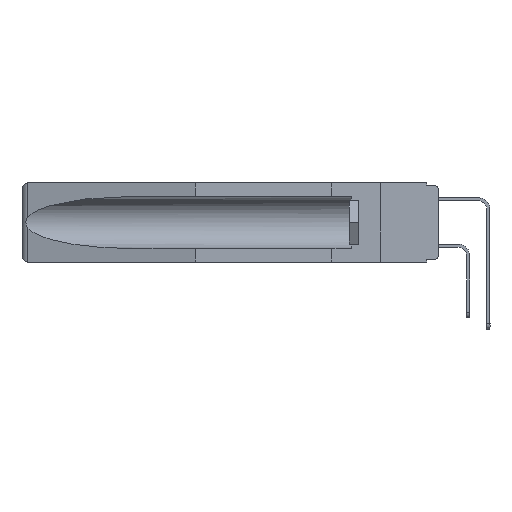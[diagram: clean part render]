
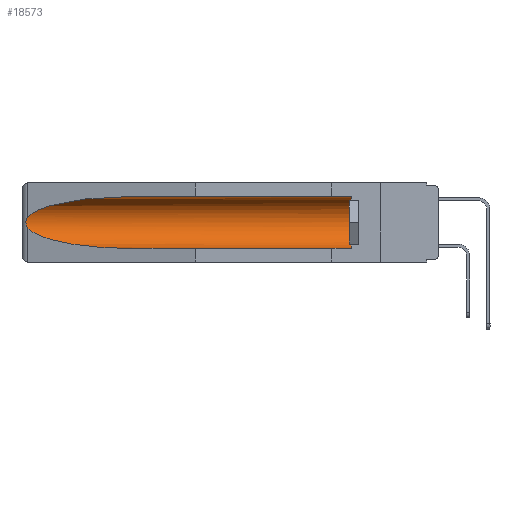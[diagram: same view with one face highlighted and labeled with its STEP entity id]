
A CAD part, left-side view. The second image highlights one B-rep face of the part: STEP entity #18573.
In plain terms, the highlighted cylindrical face has radius 2.857 mm (diameter 5.715 mm), a partial arc.
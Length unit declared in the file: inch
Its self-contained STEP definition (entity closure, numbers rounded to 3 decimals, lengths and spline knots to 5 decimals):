
#143 = VERTEX_POINT ( 'NONE', #4947 ) ;
#521 = CIRCLE ( 'NONE', #20378, 0.1125 ) ;
#637 = CARTESIAN_POINT ( 'NONE',  ( 0.155, -0.30754, -0.059 ) ) ;
#1088 = DIRECTION ( 'NONE',  ( 0., 1., 0. ) ) ;
#1167 = LINE ( 'NONE', #637, #16863 ) ;
#1213 = CARTESIAN_POINT ( 'NONE',  ( 0.155, 0.126, -0.1715 ) ) ;
#1220 = CARTESIAN_POINT ( 'NONE',  ( 0.155, -0.30754, -0.284 ) ) ;
#1757 = EDGE_CURVE ( 'NONE', #12513, #20461, #5168, .T. ) ;
#1946 = CARTESIAN_POINT ( 'NONE',  ( 0.155, 0.126, -0.284 ) ) ;
#2806 = CARTESIAN_POINT ( 'NONE',  ( 0.155, 1.07973, -0.059 ) ) ;
#3845 = CARTESIAN_POINT ( 'NONE',  ( 0.155, 0.126, -0.059 ) ) ;
#3919 = CARTESIAN_POINT ( 'NONE',  ( 0.2673, 1.5327, -0.16383 ) ) ;
#4187 = CARTESIAN_POINT ( 'NONE',  ( 0.2675, 1.53308, -0.16763 ) ) ;
#4947 = CARTESIAN_POINT ( 'NONE',  ( 0.26537, 1.52718, -0.19328 ) ) ;
#5168 = LINE ( 'NONE', #1220, #15058 ) ;
#5711 = CYLINDRICAL_SURFACE ( 'NONE', #25086, 0.1125 ) ;
#5952 = CARTESIAN_POINT ( 'NONE',  ( 0.26537, 1.52718, -0.14972 ) ) ;
#6069 = VERTEX_POINT ( 'NONE', #3845 ) ;
#6338 = CARTESIAN_POINT ( 'NONE',  ( 0.26537, 1.52718, -0.19328 ) ) ;
#6661 = EDGE_CURVE ( 'NONE', #6069, #15712, #1167, .T. ) ;
#7136 = EDGE_LOOP ( 'NONE', ( #8853, #8885, #12563, #19172, #12839, #20482 ) ) ;
#8212 = B_SPLINE_CURVE_WITH_KNOTS ( 'NONE', 3,
 ( #5952, #22687, #16041, #3919, #4187, #16575, #8360, #20645, #12142, #6338 ),
 .UNSPECIFIED., .F., .F.,
 ( 4, 2, 2, 2, 4 ),
 ( 0., 0.00029, 0.00058, 0.00087, 0.00117 ),
 .UNSPECIFIED. ) ;
#8340 = EDGE_CURVE ( 'NONE', #8698, #143, #8212, .T. ) ;
#8360 = CARTESIAN_POINT ( 'NONE',  ( 0.2673, 1.53269, -0.17917 ) ) ;
#8613 = CARTESIAN_POINT ( 'NONE',  ( 0.25451, 1.48313, -0.09465 ) ) ;
#8698 = VERTEX_POINT ( 'NONE', #25057 ) ;
#8853 = ORIENTED_EDGE ( 'NONE', *, *, #16146, .T. ) ;
#8885 = ORIENTED_EDGE ( 'NONE', *, *, #8340, .T. ) ;
#9154 = CARTESIAN_POINT ( 'NONE',  ( 0.26537, 1.52718, -0.14972 ) ) ;
#10018 = DIRECTION ( 'NONE',  ( 0., 1., 0. ) ) ;
#12142 = CARTESIAN_POINT ( 'NONE',  ( 0.26597, 1.5296, -0.19026 ) ) ;
#12513 = VERTEX_POINT ( 'NONE', #1946 ) ;
#12563 = ORIENTED_EDGE ( 'NONE', *, *, #12894, .T. ) ;
#12839 = ORIENTED_EDGE ( 'NONE', *, *, #19821, .T. ) ;
#12894 = EDGE_CURVE ( 'NONE', #143, #20461, #24536, .T. ) ;
#13246 = DIRECTION ( 'NONE',  ( 0., 0., 1. ) ) ;
#14814 = CARTESIAN_POINT ( 'NONE',  ( 0.21114, 1.30732, -0.059 ) ) ;
#15058 = VECTOR ( 'NONE', #1088, 39.37008 ) ;
#15712 = VERTEX_POINT ( 'NONE', #16884 ) ;
#16041 = CARTESIAN_POINT ( 'NONE',  ( 0.26654, 1.53092, -0.15636 ) ) ;
#16076 = FACE_OUTER_BOUND ( 'NONE', #7136, .T. ) ;
#16146 = EDGE_CURVE ( 'NONE', #15712, #8698, #17072, .T. ) ;
#16209 = DIRECTION ( 'NONE',  ( 0., 0., 1. ) ) ;
#16289 = CARTESIAN_POINT ( 'NONE',  ( 0.155, 1.07973, -0.284 ) ) ;
#16484 = CARTESIAN_POINT ( 'NONE',  ( 0.21114, 1.30732, -0.284 ) ) ;
#16575 = CARTESIAN_POINT ( 'NONE',  ( 0.2675, 1.53308, -0.17534 ) ) ;
#16863 = VECTOR ( 'NONE', #23890, 39.37008 ) ;
#16884 = CARTESIAN_POINT ( 'NONE',  ( 0.155, 1.07973, -0.059 ) ) ;
#17072 =( BOUNDED_CURVE ( )  B_SPLINE_CURVE ( 3, ( #2806, #14814, #8613, #9154 ),
 .UNSPECIFIED., .F., .F. ) 
 B_SPLINE_CURVE_WITH_KNOTS ( ( 4, 4 ),
 ( 4.71239, 6.08839 ),
 .UNSPECIFIED. ) 
 CURVE ( )  GEOMETRIC_REPRESENTATION_ITEM ( )  RATIONAL_B_SPLINE_CURVE ( ( 1., 0.848, 0.848, 1. ) ) 
 REPRESENTATION_ITEM ( '' )  );
#18397 = CARTESIAN_POINT ( 'NONE',  ( 0.155, 1.07973, -0.284 ) ) ;
#18520 = CARTESIAN_POINT ( 'NONE',  ( 0.26537, 1.52718, -0.19328 ) ) ;
#18573 = ADVANCED_FACE ( 'NONE', ( #16076 ), #5711, .F. ) ;
#19172 = ORIENTED_EDGE ( 'NONE', *, *, #1757, .F. ) ;
#19821 = EDGE_CURVE ( 'NONE', #12513, #6069, #521, .T. ) ;
#20275 = CARTESIAN_POINT ( 'NONE',  ( 0.155, -0.30754, -0.1715 ) ) ;
#20282 = CARTESIAN_POINT ( 'NONE',  ( 0.25451, 1.48313, -0.24835 ) ) ;
#20378 = AXIS2_PLACEMENT_3D ( 'NONE', #1213, #22029, #13246 ) ;
#20461 = VERTEX_POINT ( 'NONE', #16289 ) ;
#20482 = ORIENTED_EDGE ( 'NONE', *, *, #6661, .T. ) ;
#20645 = CARTESIAN_POINT ( 'NONE',  ( 0.26655, 1.53094, -0.18657 ) ) ;
#22029 = DIRECTION ( 'NONE',  ( 0., -1., 0. ) ) ;
#22687 = CARTESIAN_POINT ( 'NONE',  ( 0.26597, 1.52961, -0.15275 ) ) ;
#23890 = DIRECTION ( 'NONE',  ( 0., 1., 0. ) ) ;
#24536 =( BOUNDED_CURVE ( )  B_SPLINE_CURVE ( 3, ( #18520, #20282, #16484, #18397 ),
 .UNSPECIFIED., .F., .F. ) 
 B_SPLINE_CURVE_WITH_KNOTS ( ( 4, 4 ),
 ( 0.1948, 1.5708 ),
 .UNSPECIFIED. ) 
 CURVE ( )  GEOMETRIC_REPRESENTATION_ITEM ( )  RATIONAL_B_SPLINE_CURVE ( ( 1., 0.848, 0.848, 1. ) ) 
 REPRESENTATION_ITEM ( '' )  );
#25057 = CARTESIAN_POINT ( 'NONE',  ( 0.26537, 1.52718, -0.14972 ) ) ;
#25086 = AXIS2_PLACEMENT_3D ( 'NONE', #20275, #10018, #16209 ) ;
